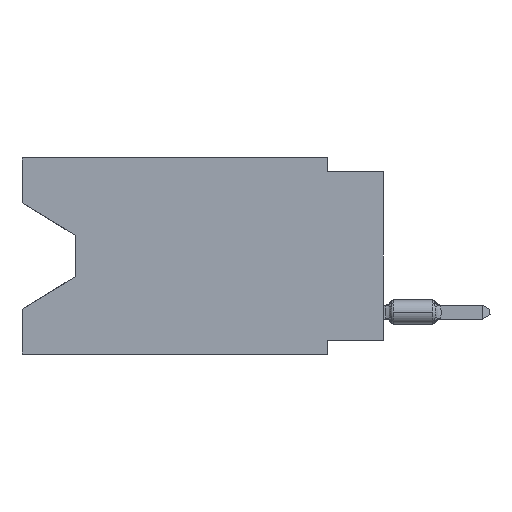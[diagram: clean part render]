
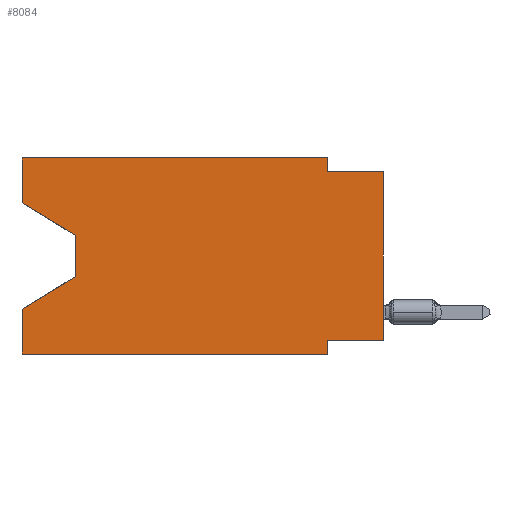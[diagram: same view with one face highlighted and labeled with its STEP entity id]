
A CAD part, left-side view. The second image highlights one B-rep face of the part: STEP entity #8084.
In plain terms, the highlighted planar face has unit normal (-1, 0, 0).
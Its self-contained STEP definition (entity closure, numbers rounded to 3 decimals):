
#132 = VERTEX_POINT ( 'NONE', #31229 ) ;
#822 = DIRECTION ( 'NONE',  ( 0., 0., 1. ) ) ;
#1230 = VECTOR ( 'NONE', #34186, 1000. ) ;
#1512 = VERTEX_POINT ( 'NONE', #19071 ) ;
#1768 = LINE ( 'NONE', #18968, #31475 ) ;
#1881 = CARTESIAN_POINT ( 'NONE',  ( 0., 2.54, 0. ) ) ;
#1882 = VECTOR ( 'NONE', #17833, 1000. ) ;
#3526 = LINE ( 'NONE', #16980, #1230 ) ;
#3824 = EDGE_CURVE ( 'NONE', #27817, #14330, #42034, .T. ) ;
#4966 = LINE ( 'NONE', #11780, #42364 ) ;
#5077 = EDGE_CURVE ( 'NONE', #23004, #27817, #3526, .T. ) ;
#6233 = CARTESIAN_POINT ( 'NONE',  ( 0., 16.383, -2.038 ) ) ;
#6542 = EDGE_LOOP ( 'NONE', ( #19912, #31167, #22981, #22351, #42699, #36859, #14765, #16991, #35821, #9853, #28417, #34169 ) ) ;
#6562 = VERTEX_POINT ( 'NONE', #10597 ) ;
#7590 = CARTESIAN_POINT ( 'NONE',  ( 0., 16.383, -6.852 ) ) ;
#8084 = ADVANCED_FACE ( 'NONE', ( #17855 ), #31302, .F. ) ;
#9853 = ORIENTED_EDGE ( 'NONE', *, *, #36143, .F. ) ;
#10381 = CARTESIAN_POINT ( 'NONE',  ( 0., 16.383, -8.89 ) ) ;
#10597 = CARTESIAN_POINT ( 'NONE',  ( 0., 0., -0.635 ) ) ;
#10939 = CARTESIAN_POINT ( 'NONE',  ( 0., 16.383, 0. ) ) ;
#11780 = CARTESIAN_POINT ( 'NONE',  ( 0., 2.54, -8.89 ) ) ;
#12903 = DIRECTION ( 'NONE',  ( 0., -1., 0. ) ) ;
#13761 = LINE ( 'NONE', #37619, #32790 ) ;
#14140 = EDGE_CURVE ( 'NONE', #1512, #6562, #13761, .T. ) ;
#14330 = VERTEX_POINT ( 'NONE', #7590 ) ;
#14426 = VERTEX_POINT ( 'NONE', #6233 ) ;
#14527 = CARTESIAN_POINT ( 'NONE',  ( 0., 16.383, 0. ) ) ;
#14765 = ORIENTED_EDGE ( 'NONE', *, *, #15415, .F. ) ;
#15415 = EDGE_CURVE ( 'NONE', #18874, #36978, #31085, .T. ) ;
#15664 = VERTEX_POINT ( 'NONE', #40983 ) ;
#15667 = CARTESIAN_POINT ( 'NONE',  ( 0., 13.97, -5.385 ) ) ;
#16224 = AXIS2_PLACEMENT_3D ( 'NONE', #14527, #21370, #28001 ) ;
#16810 = VECTOR ( 'NONE', #12903, 1000. ) ;
#16980 = CARTESIAN_POINT ( 'NONE',  ( 0., 13.97, -3.505 ) ) ;
#16991 = ORIENTED_EDGE ( 'NONE', *, *, #22258, .T. ) ;
#17085 = DIRECTION ( 'NONE',  ( 0., -1., 0. ) ) ;
#17833 = DIRECTION ( 'NONE',  ( 0., 1., 0. ) ) ;
#17855 = FACE_OUTER_BOUND ( 'NONE', #6542, .T. ) ;
#18123 = VECTOR ( 'NONE', #42283, 1000. ) ;
#18536 = DIRECTION ( 'NONE',  ( 0., 0., 1. ) ) ;
#18708 = EDGE_CURVE ( 'NONE', #35618, #14330, #31036, .T. ) ;
#18874 = VERTEX_POINT ( 'NONE', #22850 ) ;
#18968 = CARTESIAN_POINT ( 'NONE',  ( 0., 16.383, 0. ) ) ;
#19071 = CARTESIAN_POINT ( 'NONE',  ( 0., 2.54, -0.635 ) ) ;
#19496 = CARTESIAN_POINT ( 'NONE',  ( 0., 13.97, -5.385 ) ) ;
#19745 = LINE ( 'NONE', #40074, #16810 ) ;
#19912 = ORIENTED_EDGE ( 'NONE', *, *, #32983, .T. ) ;
#20035 = CARTESIAN_POINT ( 'NONE',  ( 0., 0., -8.255 ) ) ;
#20296 = DIRECTION ( 'NONE',  ( 0., -1., 0. ) ) ;
#21370 = DIRECTION ( 'NONE',  ( 1., 0., 0. ) ) ;
#22258 = EDGE_CURVE ( 'NONE', #18874, #6562, #42365, .T. ) ;
#22351 = ORIENTED_EDGE ( 'NONE', *, *, #18708, .F. ) ;
#22850 = CARTESIAN_POINT ( 'NONE',  ( 0., 0., -8.255 ) ) ;
#22898 = CARTESIAN_POINT ( 'NONE',  ( 0., 2.54, -8.89 ) ) ;
#22981 = ORIENTED_EDGE ( 'NONE', *, *, #3824, .T. ) ;
#23004 = VERTEX_POINT ( 'NONE', #35412 ) ;
#24743 = VECTOR ( 'NONE', #822, 1000. ) ;
#25382 = EDGE_CURVE ( 'NONE', #35618, #40235, #37738, .T. ) ;
#27817 = VERTEX_POINT ( 'NONE', #15667 ) ;
#28001 = DIRECTION ( 'NONE',  ( 0., 0., -1. ) ) ;
#28417 = ORIENTED_EDGE ( 'NONE', *, *, #37368, .F. ) ;
#30292 = CARTESIAN_POINT ( 'NONE',  ( 0., 16.383, -2.038 ) ) ;
#31036 = LINE ( 'NONE', #10939, #24743 ) ;
#31085 = LINE ( 'NONE', #20035, #1882 ) ;
#31167 = ORIENTED_EDGE ( 'NONE', *, *, #5077, .T. ) ;
#31229 = CARTESIAN_POINT ( 'NONE',  ( 0., 16.383, 0. ) ) ;
#31302 = PLANE ( 'NONE',  #16224 ) ;
#31424 = DIRECTION ( 'NONE',  ( 0., 0., -1. ) ) ;
#31475 = VECTOR ( 'NONE', #18536, 1000. ) ;
#32637 = DIRECTION ( 'NONE',  ( 0., 0., 1. ) ) ;
#32790 = VECTOR ( 'NONE', #17085, 1000. ) ;
#32983 = EDGE_CURVE ( 'NONE', #14426, #23004, #37136, .T. ) ;
#33131 = VECTOR ( 'NONE', #32637, 1000. ) ;
#33726 = CARTESIAN_POINT ( 'NONE',  ( 0., 2.54, -8.255 ) ) ;
#34169 = ORIENTED_EDGE ( 'NONE', *, *, #35403, .F. ) ;
#34186 = DIRECTION ( 'NONE',  ( 0., 0., -1. ) ) ;
#35403 = EDGE_CURVE ( 'NONE', #14426, #132, #1768, .T. ) ;
#35412 = CARTESIAN_POINT ( 'NONE',  ( 0., 13.97, -3.505 ) ) ;
#35618 = VERTEX_POINT ( 'NONE', #41693 ) ;
#35821 = ORIENTED_EDGE ( 'NONE', *, *, #14140, .F. ) ;
#36143 = EDGE_CURVE ( 'NONE', #15664, #1512, #42702, .T. ) ;
#36287 = VECTOR ( 'NONE', #40664, 1000. ) ;
#36859 = ORIENTED_EDGE ( 'NONE', *, *, #40865, .F. ) ;
#36978 = VERTEX_POINT ( 'NONE', #33726 ) ;
#37037 = VECTOR ( 'NONE', #20296, 1000. ) ;
#37136 = LINE ( 'NONE', #30292, #36287 ) ;
#37368 = EDGE_CURVE ( 'NONE', #132, #15664, #19745, .T. ) ;
#37619 = CARTESIAN_POINT ( 'NONE',  ( 0., 0., -0.635 ) ) ;
#37738 = LINE ( 'NONE', #10381, #37037 ) ;
#39151 = DIRECTION ( 'NONE',  ( 0., 0.855, -0.519 ) ) ;
#39180 = VECTOR ( 'NONE', #39151, 1000. ) ;
#40074 = CARTESIAN_POINT ( 'NONE',  ( 0., 16.383, 0. ) ) ;
#40235 = VERTEX_POINT ( 'NONE', #22898 ) ;
#40664 = DIRECTION ( 'NONE',  ( 0., -0.855, -0.519 ) ) ;
#40865 = EDGE_CURVE ( 'NONE', #36978, #40235, #4966, .T. ) ;
#40983 = CARTESIAN_POINT ( 'NONE',  ( 0., 2.54, 0. ) ) ;
#41693 = CARTESIAN_POINT ( 'NONE',  ( 0., 16.383, -8.89 ) ) ;
#42034 = LINE ( 'NONE', #19496, #39180 ) ;
#42149 = CARTESIAN_POINT ( 'NONE',  ( 0., 0., 0. ) ) ;
#42283 = DIRECTION ( 'NONE',  ( 0., 0., -1. ) ) ;
#42364 = VECTOR ( 'NONE', #31424, 1000. ) ;
#42365 = LINE ( 'NONE', #42149, #33131 ) ;
#42699 = ORIENTED_EDGE ( 'NONE', *, *, #25382, .T. ) ;
#42702 = LINE ( 'NONE', #1881, #18123 ) ;
